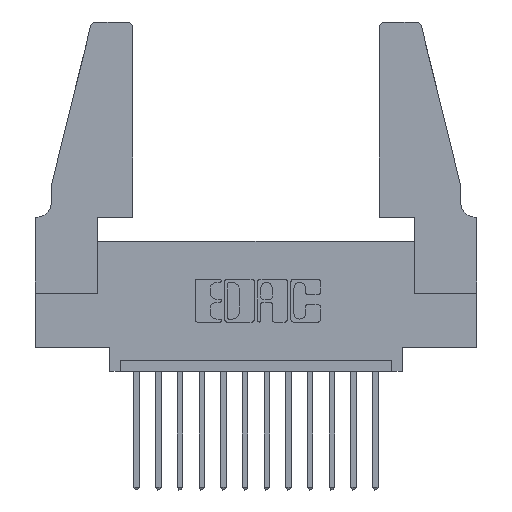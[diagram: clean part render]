
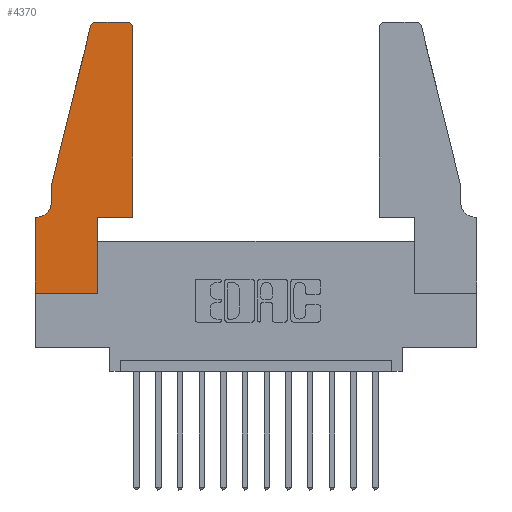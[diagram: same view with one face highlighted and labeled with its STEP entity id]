
A CAD part, top view. The second image highlights one B-rep face of the part: STEP entity #4370.
In plain terms, the highlighted planar face has unit normal (0, 0, 1).
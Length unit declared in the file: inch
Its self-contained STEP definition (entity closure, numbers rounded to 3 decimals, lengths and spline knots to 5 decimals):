
#186 = VERTEX_POINT ( 'NONE', #9423 ) ;
#239 = DIRECTION ( 'NONE',  ( 1., 0., 0. ) ) ;
#297 = VERTEX_POINT ( 'NONE', #1670 ) ;
#352 = EDGE_CURVE ( 'NONE', #3694, #2223, #3682, .T. ) ;
#411 = VECTOR ( 'NONE', #13320, 39.37008 ) ;
#599 = CARTESIAN_POINT ( 'NONE',  ( 0.25487, 1.22718, 0.37 ) ) ;
#662 = FACE_OUTER_BOUND ( 'NONE', #4590, .T. ) ;
#688 = VERTEX_POINT ( 'NONE', #5603 ) ;
#722 = ORIENTED_EDGE ( 'NONE', *, *, #352, .T. ) ;
#774 = AXIS2_PLACEMENT_3D ( 'NONE', #3798, #7332, #239 ) ;
#778 = VECTOR ( 'NONE', #1229, 39.37008 ) ;
#1229 = DIRECTION ( 'NONE',  ( 0., 1., 0. ) ) ;
#1277 = VERTEX_POINT ( 'NONE', #14033 ) ;
#1446 = ORIENTED_EDGE ( 'NONE', *, *, #8420, .T. ) ;
#1461 = CARTESIAN_POINT ( 'NONE',  ( 0.0055, 0.42, 0.37 ) ) ;
#1465 = EDGE_CURVE ( 'NONE', #14041, #297, #6378, .T. ) ;
#1526 = CIRCLE ( 'NONE', #774, 0.03 ) ;
#1670 = CARTESIAN_POINT ( 'NONE',  ( 0.4505, 0.35, 0.37 ) ) ;
#1711 = VERTEX_POINT ( 'NONE', #6642 ) ;
#1851 = VECTOR ( 'NONE', #5414, 39.37008 ) ;
#1862 = EDGE_CURVE ( 'NONE', #1711, #13534, #9852, .T. ) ;
#2028 = EDGE_CURVE ( 'NONE', #13534, #4949, #6732, .T. ) ;
#2223 = VERTEX_POINT ( 'NONE', #11969 ) ;
#2518 = LINE ( 'NONE', #15200, #5301 ) ;
#2681 = CARTESIAN_POINT ( 'NONE',  ( 0.2605, 1.25, 0.37 ) ) ;
#3039 = CARTESIAN_POINT ( 'NONE',  ( 0.0755, 0.5, 0.37 ) ) ;
#3359 = ORIENTED_EDGE ( 'NONE', *, *, #9087, .T. ) ;
#3423 = LINE ( 'NONE', #3487, #778 ) ;
#3487 = CARTESIAN_POINT ( 'NONE',  ( 0.4505, 0.35, 0.37 ) ) ;
#3624 = LINE ( 'NONE', #2681, #411 ) ;
#3682 = LINE ( 'NONE', #11042, #6782 ) ;
#3694 = VERTEX_POINT ( 'NONE', #599 ) ;
#3727 = CARTESIAN_POINT ( 'NONE',  ( 0., 0., 0.37 ) ) ;
#3798 = CARTESIAN_POINT ( 'NONE',  ( 0.4205, 1.22, 0.37 ) ) ;
#3812 = CARTESIAN_POINT ( 'NONE',  ( 0.0755, 0.35, 0.37 ) ) ;
#4064 = CARTESIAN_POINT ( 'NONE',  ( 0., 0.35, 0.37 ) ) ;
#4370 = ADVANCED_FACE ( 'NONE', ( #662 ), #14699, .T. ) ;
#4521 = ORIENTED_EDGE ( 'NONE', *, *, #1862, .T. ) ;
#4575 = DIRECTION ( 'NONE',  ( -1., 0., 0. ) ) ;
#4590 = EDGE_LOOP ( 'NONE', ( #9178, #15363, #722, #3359, #10672, #4521, #8953, #1446, #5150, #5200, #5035, #5762 ) ) ;
#4935 = EDGE_CURVE ( 'NONE', #1277, #1711, #6944, .T. ) ;
#4949 = VERTEX_POINT ( 'NONE', #3727 ) ;
#5035 = ORIENTED_EDGE ( 'NONE', *, *, #6049, .T. ) ;
#5145 = CARTESIAN_POINT ( 'NONE',  ( 0., 0., 0.37 ) ) ;
#5150 = ORIENTED_EDGE ( 'NONE', *, *, #14469, .T. ) ;
#5200 = ORIENTED_EDGE ( 'NONE', *, *, #1465, .T. ) ;
#5273 = CARTESIAN_POINT ( 'NONE',  ( 0., 0.35, 0.37 ) ) ;
#5301 = VECTOR ( 'NONE', #5821, 39.37008 ) ;
#5372 = VECTOR ( 'NONE', #10061, 39.37008 ) ;
#5414 = DIRECTION ( 'NONE',  ( 1., 0., 0. ) ) ;
#5444 = CARTESIAN_POINT ( 'NONE',  ( 0.284, 1.22, 0.37 ) ) ;
#5603 = CARTESIAN_POINT ( 'NONE',  ( 0.4505, 1.22, 0.37 ) ) ;
#5762 = ORIENTED_EDGE ( 'NONE', *, *, #5940, .T. ) ;
#5821 = DIRECTION ( 'NONE',  ( 0., 1., 0. ) ) ;
#5891 = AXIS2_PLACEMENT_3D ( 'NONE', #5444, #6599, #7770 ) ;
#5940 = EDGE_CURVE ( 'NONE', #688, #186, #1526, .T. ) ;
#6049 = EDGE_CURVE ( 'NONE', #297, #688, #3423, .T. ) ;
#6378 = LINE ( 'NONE', #13100, #13051 ) ;
#6411 = DIRECTION ( 'NONE',  ( 1., 0., 0. ) ) ;
#6495 = EDGE_CURVE ( 'NONE', #186, #14582, #3624, .T. ) ;
#6511 = DIRECTION ( 'NONE',  ( 0., 0., 1. ) ) ;
#6599 = DIRECTION ( 'NONE',  ( 0., 0., 1. ) ) ;
#6642 = CARTESIAN_POINT ( 'NONE',  ( 0.0055, 0.35, 0.37 ) ) ;
#6732 = LINE ( 'NONE', #13513, #12660 ) ;
#6782 = VECTOR ( 'NONE', #7397, 39.37008 ) ;
#6944 = CIRCLE ( 'NONE', #13275, 0.07 ) ;
#7201 = DIRECTION ( 'NONE',  ( 1., 0., 0. ) ) ;
#7332 = DIRECTION ( 'NONE',  ( 0., 0., 1. ) ) ;
#7397 = DIRECTION ( 'NONE',  ( -0.239, -0.971, 0. ) ) ;
#7770 = DIRECTION ( 'NONE',  ( 1., 0., 0. ) ) ;
#8420 = EDGE_CURVE ( 'NONE', #4949, #10197, #14446, .T. ) ;
#8582 = CARTESIAN_POINT ( 'NONE',  ( 0.2865, 0.35, 0.37 ) ) ;
#8953 = ORIENTED_EDGE ( 'NONE', *, *, #2028, .T. ) ;
#9087 = EDGE_CURVE ( 'NONE', #2223, #1277, #9414, .T. ) ;
#9178 = ORIENTED_EDGE ( 'NONE', *, *, #6495, .T. ) ;
#9414 = LINE ( 'NONE', #3039, #5372 ) ;
#9423 = CARTESIAN_POINT ( 'NONE',  ( 0.4205, 1.25, 0.37 ) ) ;
#9515 = CARTESIAN_POINT ( 'NONE',  ( 0.284, 1.25, 0.37 ) ) ;
#9716 = DIRECTION ( 'NONE',  ( 0., 0., -1. ) ) ;
#9852 = LINE ( 'NONE', #3812, #12273 ) ;
#9876 = AXIS2_PLACEMENT_3D ( 'NONE', #4064, #6511, #6411 ) ;
#10032 = DIRECTION ( 'NONE',  ( 0., -1., 0. ) ) ;
#10061 = DIRECTION ( 'NONE',  ( 0., -1., 0. ) ) ;
#10195 = CIRCLE ( 'NONE', #5891, 0.03 ) ;
#10197 = VERTEX_POINT ( 'NONE', #15344 ) ;
#10672 = ORIENTED_EDGE ( 'NONE', *, *, #4935, .T. ) ;
#11042 = CARTESIAN_POINT ( 'NONE',  ( 0.0755, 0.5, 0.37 ) ) ;
#11124 = EDGE_CURVE ( 'NONE', #14582, #3694, #10195, .T. ) ;
#11969 = CARTESIAN_POINT ( 'NONE',  ( 0.0755, 0.5, 0.37 ) ) ;
#12071 = DIRECTION ( 'NONE',  ( -1., 0., 0. ) ) ;
#12273 = VECTOR ( 'NONE', #4575, 39.37008 ) ;
#12660 = VECTOR ( 'NONE', #10032, 39.37008 ) ;
#13051 = VECTOR ( 'NONE', #7201, 39.37008 ) ;
#13100 = CARTESIAN_POINT ( 'NONE',  ( 0.4505, 0.35, 0.37 ) ) ;
#13275 = AXIS2_PLACEMENT_3D ( 'NONE', #1461, #9716, #12071 ) ;
#13320 = DIRECTION ( 'NONE',  ( -1., 0., 0. ) ) ;
#13513 = CARTESIAN_POINT ( 'NONE',  ( 0., 0., 0.37 ) ) ;
#13534 = VERTEX_POINT ( 'NONE', #5273 ) ;
#14033 = CARTESIAN_POINT ( 'NONE',  ( 0.0755, 0.42, 0.37 ) ) ;
#14041 = VERTEX_POINT ( 'NONE', #8582 ) ;
#14446 = LINE ( 'NONE', #5145, #1851 ) ;
#14469 = EDGE_CURVE ( 'NONE', #10197, #14041, #2518, .T. ) ;
#14582 = VERTEX_POINT ( 'NONE', #9515 ) ;
#14699 = PLANE ( 'NONE',  #9876 ) ;
#15200 = CARTESIAN_POINT ( 'NONE',  ( 0.2865, 0.35, 0.37 ) ) ;
#15344 = CARTESIAN_POINT ( 'NONE',  ( 0.2865, 0., 0.37 ) ) ;
#15363 = ORIENTED_EDGE ( 'NONE', *, *, #11124, .T. ) ;
